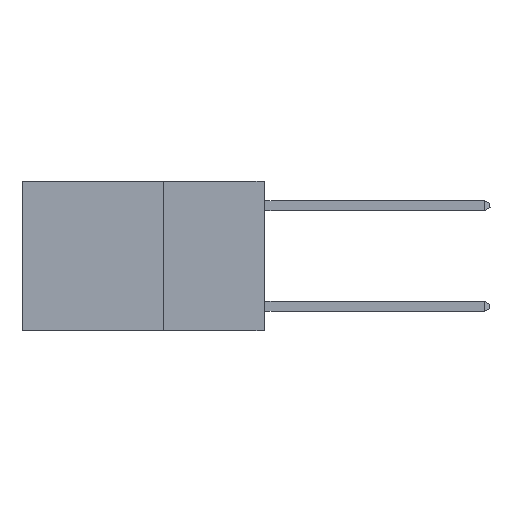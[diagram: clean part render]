
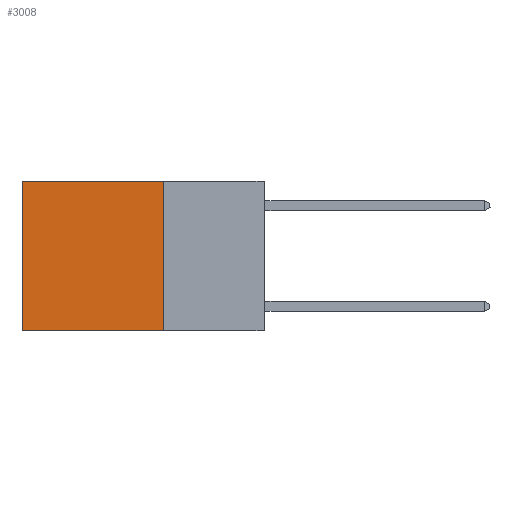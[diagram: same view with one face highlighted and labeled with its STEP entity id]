
A CAD part, left-side view. The second image highlights one B-rep face of the part: STEP entity #3008.
In plain terms, the highlighted planar face has unit normal (-1, 0, 0).
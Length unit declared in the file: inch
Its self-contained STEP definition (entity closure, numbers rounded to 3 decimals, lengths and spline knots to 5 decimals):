
#409 = VERTEX_POINT ( 'NONE', #9987 ) ;
#786 = CARTESIAN_POINT ( 'NONE',  ( 0.2625, 0.25, 0. ) ) ;
#1486 = CARTESIAN_POINT ( 'NONE',  ( 0.2625, 0.25, -0.37 ) ) ;
#1949 = CARTESIAN_POINT ( 'NONE',  ( 0.2625, 0.6, 0. ) ) ;
#1984 = VECTOR ( 'NONE', #4725, 39.37008 ) ;
#2310 = VERTEX_POINT ( 'NONE', #12648 ) ;
#2463 = CARTESIAN_POINT ( 'NONE',  ( 0.2625, 0.6, 0. ) ) ;
#2745 = VERTEX_POINT ( 'NONE', #2463 ) ;
#3008 = ADVANCED_FACE ( 'NONE', ( #5356 ), #4364, .F. ) ;
#3078 = EDGE_CURVE ( 'NONE', #2310, #409, #12566, .T. ) ;
#3404 = DIRECTION ( 'NONE',  ( 0., 0., -1. ) ) ;
#3598 = DIRECTION ( 'NONE',  ( 0., 1., 0. ) ) ;
#4364 = PLANE ( 'NONE',  #9535 ) ;
#4725 = DIRECTION ( 'NONE',  ( 0., 0., -1. ) ) ;
#5356 = FACE_OUTER_BOUND ( 'NONE', #11935, .T. ) ;
#5785 = LINE ( 'NONE', #786, #1984 ) ;
#5806 = VECTOR ( 'NONE', #10970, 39.37008 ) ;
#6163 = LINE ( 'NONE', #9900, #5806 ) ;
#6534 = ORIENTED_EDGE ( 'NONE', *, *, #8307, .F. ) ;
#6910 = LINE ( 'NONE', #1949, #11462 ) ;
#7292 = VERTEX_POINT ( 'NONE', #9177 ) ;
#7451 = VECTOR ( 'NONE', #3598, 39.37008 ) ;
#7676 = DIRECTION ( 'NONE',  ( 0., 0., -1. ) ) ;
#8307 = EDGE_CURVE ( 'NONE', #7292, #2310, #5785, .T. ) ;
#9177 = CARTESIAN_POINT ( 'NONE',  ( 0.2625, 0.25, 0. ) ) ;
#9535 = AXIS2_PLACEMENT_3D ( 'NONE', #12116, #11155, #3404 ) ;
#9707 = EDGE_CURVE ( 'NONE', #2745, #409, #6910, .T. ) ;
#9840 = ORIENTED_EDGE ( 'NONE', *, *, #10679, .T. ) ;
#9900 = CARTESIAN_POINT ( 'NONE',  ( 0.2625, 0.25, 0. ) ) ;
#9987 = CARTESIAN_POINT ( 'NONE',  ( 0.2625, 0.6, -0.37 ) ) ;
#10679 = EDGE_CURVE ( 'NONE', #7292, #2745, #6163, .T. ) ;
#10951 = ORIENTED_EDGE ( 'NONE', *, *, #3078, .F. ) ;
#10970 = DIRECTION ( 'NONE',  ( 0., 1., 0. ) ) ;
#11155 = DIRECTION ( 'NONE',  ( 1., 0., 0. ) ) ;
#11462 = VECTOR ( 'NONE', #7676, 39.37008 ) ;
#11935 = EDGE_LOOP ( 'NONE', ( #12536, #10951, #6534, #9840 ) ) ;
#12116 = CARTESIAN_POINT ( 'NONE',  ( 0.2625, 0.25, 0. ) ) ;
#12536 = ORIENTED_EDGE ( 'NONE', *, *, #9707, .T. ) ;
#12566 = LINE ( 'NONE', #1486, #7451 ) ;
#12648 = CARTESIAN_POINT ( 'NONE',  ( 0.2625, 0.25, -0.37 ) ) ;
